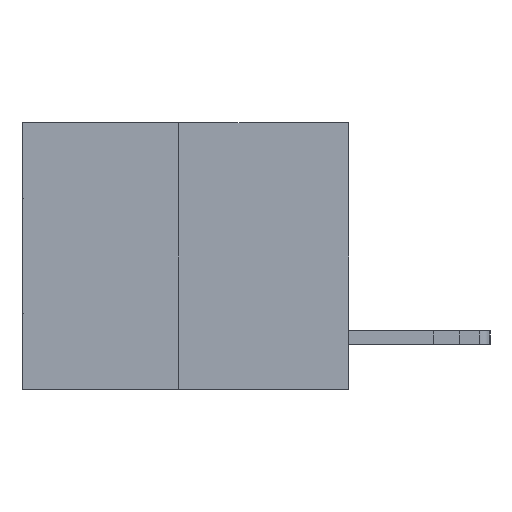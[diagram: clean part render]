
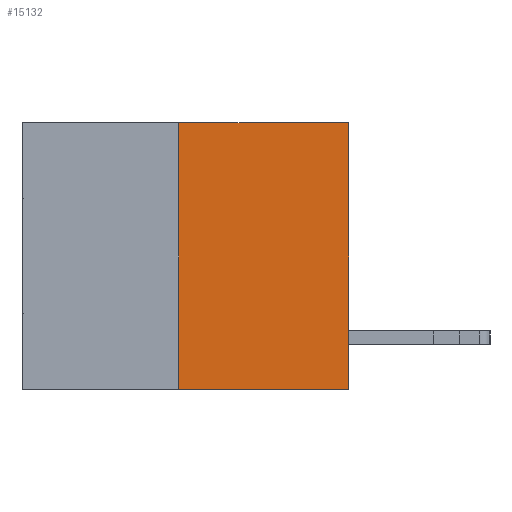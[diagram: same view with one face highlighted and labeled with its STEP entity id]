
A CAD part, left-side view. The second image highlights one B-rep face of the part: STEP entity #15132.
In plain terms, the highlighted planar face has unit normal (-1, 0, 0).
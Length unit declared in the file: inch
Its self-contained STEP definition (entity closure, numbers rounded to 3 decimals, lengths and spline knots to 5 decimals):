
#37 = EDGE_LOOP ( 'NONE', ( #20852, #25960, #14443, #4655 ) ) ;
#772 = CARTESIAN_POINT ( 'NONE',  ( 0., 0.6, -0.49 ) ) ;
#898 = EDGE_CURVE ( 'NONE', #25108, #26152, #27098, .T. ) ;
#1617 = CARTESIAN_POINT ( 'NONE',  ( 0., 0.6, 0. ) ) ;
#1952 = LINE ( 'NONE', #3076, #16068 ) ;
#1969 = VERTEX_POINT ( 'NONE', #29355 ) ;
#3076 = CARTESIAN_POINT ( 'NONE',  ( 0., 0.6, 0. ) ) ;
#3786 = CARTESIAN_POINT ( 'NONE',  ( 0., 0., -0.49 ) ) ;
#3991 = DIRECTION ( 'NONE',  ( 1., 0., 0. ) ) ;
#4655 = ORIENTED_EDGE ( 'NONE', *, *, #20659, .F. ) ;
#4774 = CARTESIAN_POINT ( 'NONE',  ( 0., 0.312, 0. ) ) ;
#4888 = CARTESIAN_POINT ( 'NONE',  ( 0., 0., 0. ) ) ;
#6504 = EDGE_CURVE ( 'NONE', #25108, #6505, #15488, .T. ) ;
#6505 = VERTEX_POINT ( 'NONE', #4774 ) ;
#7866 = LINE ( 'NONE', #4888, #29711 ) ;
#8331 = FACE_OUTER_BOUND ( 'NONE', #37, .T. ) ;
#9029 = EDGE_CURVE ( 'NONE', #26152, #1969, #7866, .T. ) ;
#10112 = DIRECTION ( 'NONE',  ( 0., 0., 1. ) ) ;
#11742 = CARTESIAN_POINT ( 'NONE',  ( 0., 0.312, -0.49 ) ) ;
#13097 = CARTESIAN_POINT ( 'NONE',  ( 0., 0.312, -0.49 ) ) ;
#13124 = DIRECTION ( 'NONE',  ( 0., -1., 0. ) ) ;
#13768 = VECTOR ( 'NONE', #19544, 39.37008 ) ;
#14443 = ORIENTED_EDGE ( 'NONE', *, *, #9029, .T. ) ;
#15132 = ADVANCED_FACE ( 'NONE', ( #8331 ), #18092, .F. ) ;
#15488 = LINE ( 'NONE', #11742, #22503 ) ;
#16068 = VECTOR ( 'NONE', #13124, 39.37008 ) ;
#18092 = PLANE ( 'NONE',  #26132 ) ;
#19544 = DIRECTION ( 'NONE',  ( 0., -1., 0. ) ) ;
#20659 = EDGE_CURVE ( 'NONE', #6505, #1969, #1952, .T. ) ;
#20852 = ORIENTED_EDGE ( 'NONE', *, *, #6504, .F. ) ;
#22503 = VECTOR ( 'NONE', #30544, 39.37008 ) ;
#22550 = DIRECTION ( 'NONE',  ( 0., 0., -1. ) ) ;
#25108 = VERTEX_POINT ( 'NONE', #13097 ) ;
#25960 = ORIENTED_EDGE ( 'NONE', *, *, #898, .T. ) ;
#26132 = AXIS2_PLACEMENT_3D ( 'NONE', #1617, #3991, #22550 ) ;
#26152 = VERTEX_POINT ( 'NONE', #3786 ) ;
#27098 = LINE ( 'NONE', #772, #13768 ) ;
#29355 = CARTESIAN_POINT ( 'NONE',  ( 0., 0., 0. ) ) ;
#29711 = VECTOR ( 'NONE', #10112, 39.37008 ) ;
#30544 = DIRECTION ( 'NONE',  ( 0., 0., 1. ) ) ;
